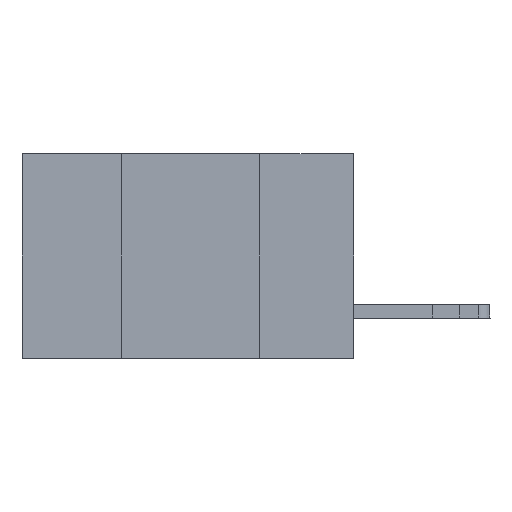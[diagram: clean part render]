
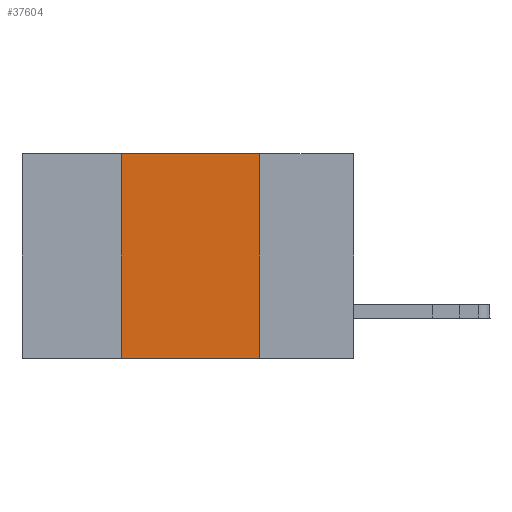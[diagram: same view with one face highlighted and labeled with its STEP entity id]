
A CAD part, left-side view. The second image highlights one B-rep face of the part: STEP entity #37604.
In plain terms, the highlighted planar face has unit normal (-1, 0, 0).
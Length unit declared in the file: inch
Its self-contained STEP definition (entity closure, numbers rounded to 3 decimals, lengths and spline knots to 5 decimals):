
#194 = EDGE_CURVE ( 'NONE', #36795, #25103, #17869, .T. ) ;
#234 = EDGE_CURVE ( 'NONE', #2664, #8654, #34053, .T. ) ;
#1044 = CARTESIAN_POINT ( 'NONE',  ( 0., 0.17, 0. ) ) ;
#1319 = CARTESIAN_POINT ( 'NONE',  ( 0., 0.6, 0. ) ) ;
#2664 = VERTEX_POINT ( 'NONE', #1044 ) ;
#4496 = CARTESIAN_POINT ( 'NONE',  ( 0., 0.6, -0.37 ) ) ;
#5788 = CARTESIAN_POINT ( 'NONE',  ( 0., 0.42, 0. ) ) ;
#7667 = LINE ( 'NONE', #4496, #28588 ) ;
#8546 = EDGE_LOOP ( 'NONE', ( #32272, #30133, #33669, #18291 ) ) ;
#8654 = VERTEX_POINT ( 'NONE', #16105 ) ;
#11063 = CARTESIAN_POINT ( 'NONE',  ( 0., 0.6, 0. ) ) ;
#11274 = EDGE_CURVE ( 'NONE', #25103, #2664, #31025, .T. ) ;
#12140 = VECTOR ( 'NONE', #34175, 39.37008 ) ;
#12507 = DIRECTION ( 'NONE',  ( 0., 0., -1. ) ) ;
#14226 = VECTOR ( 'NONE', #18059, 39.37008 ) ;
#14412 = PLANE ( 'NONE',  #20045 ) ;
#15526 = VECTOR ( 'NONE', #12507, 39.37008 ) ;
#15661 = CARTESIAN_POINT ( 'NONE',  ( 0., 0.17, 0. ) ) ;
#16105 = CARTESIAN_POINT ( 'NONE',  ( 0., 0.17, -0.37 ) ) ;
#16371 = DIRECTION ( 'NONE',  ( 0., -1., 0. ) ) ;
#17869 = LINE ( 'NONE', #5788, #14226 ) ;
#18059 = DIRECTION ( 'NONE',  ( 0., 0., 1. ) ) ;
#18291 = ORIENTED_EDGE ( 'NONE', *, *, #24237, .T. ) ;
#20045 = AXIS2_PLACEMENT_3D ( 'NONE', #11063, #23133, #26494 ) ;
#21324 = CARTESIAN_POINT ( 'NONE',  ( 0., 0.42, -0.37 ) ) ;
#23133 = DIRECTION ( 'NONE',  ( 1., 0., 0. ) ) ;
#24237 = EDGE_CURVE ( 'NONE', #36795, #8654, #7667, .T. ) ;
#25103 = VERTEX_POINT ( 'NONE', #35921 ) ;
#26494 = DIRECTION ( 'NONE',  ( 0., 0., -1. ) ) ;
#28588 = VECTOR ( 'NONE', #16371, 39.37008 ) ;
#30133 = ORIENTED_EDGE ( 'NONE', *, *, #11274, .F. ) ;
#31025 = LINE ( 'NONE', #1319, #12140 ) ;
#32272 = ORIENTED_EDGE ( 'NONE', *, *, #234, .F. ) ;
#33669 = ORIENTED_EDGE ( 'NONE', *, *, #194, .F. ) ;
#34053 = LINE ( 'NONE', #15661, #15526 ) ;
#34175 = DIRECTION ( 'NONE',  ( 0., -1., 0. ) ) ;
#35202 = FACE_OUTER_BOUND ( 'NONE', #8546, .T. ) ;
#35921 = CARTESIAN_POINT ( 'NONE',  ( 0., 0.42, 0. ) ) ;
#36795 = VERTEX_POINT ( 'NONE', #21324 ) ;
#37604 = ADVANCED_FACE ( 'NONE', ( #35202 ), #14412, .F. ) ;
